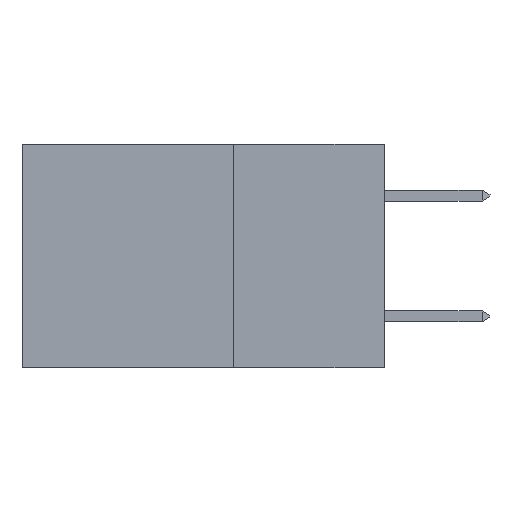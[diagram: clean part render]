
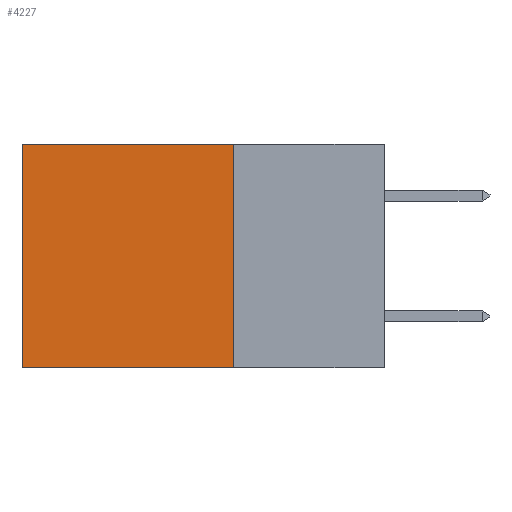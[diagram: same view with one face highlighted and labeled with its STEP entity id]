
A CAD part, left-side view. The second image highlights one B-rep face of the part: STEP entity #4227.
In plain terms, the highlighted planar face has unit normal (-1, 0, 0).
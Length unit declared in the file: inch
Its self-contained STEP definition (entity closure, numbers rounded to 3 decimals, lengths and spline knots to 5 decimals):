
#664 = LINE ( 'NONE', #10411, #8537 ) ;
#1403 = VERTEX_POINT ( 'NONE', #13510 ) ;
#2851 = DIRECTION ( 'NONE',  ( 0., 1., 0. ) ) ;
#2988 = VECTOR ( 'NONE', #2851, 39.37008 ) ;
#3219 = CARTESIAN_POINT ( 'NONE',  ( 0.2875, 0.25, -0.37 ) ) ;
#3693 = CARTESIAN_POINT ( 'NONE',  ( 0.2875, 0.6, -0.37 ) ) ;
#3797 = DIRECTION ( 'NONE',  ( 0., 0., -1. ) ) ;
#3848 = DIRECTION ( 'NONE',  ( 1., 0., 0. ) ) ;
#3862 = PLANE ( 'NONE',  #3937 ) ;
#3937 = AXIS2_PLACEMENT_3D ( 'NONE', #3963, #3848, #3797 ) ;
#3963 = CARTESIAN_POINT ( 'NONE',  ( 0.2875, 0.25, 0. ) ) ;
#3998 = EDGE_CURVE ( 'NONE', #10174, #11078, #10916, .T. ) ;
#4227 = ADVANCED_FACE ( 'NONE', ( #15307 ), #3862, .F. ) ;
#4277 = EDGE_CURVE ( 'NONE', #1403, #11078, #7198, .T. ) ;
#6881 = ORIENTED_EDGE ( 'NONE', *, *, #18691, .T. ) ;
#6943 = ORIENTED_EDGE ( 'NONE', *, *, #10071, .F. ) ;
#7198 = LINE ( 'NONE', #3219, #2988 ) ;
#7829 = DIRECTION ( 'NONE',  ( 0., 0., -1. ) ) ;
#7894 = CARTESIAN_POINT ( 'NONE',  ( 0.2875, 0.6, 0. ) ) ;
#8327 = VECTOR ( 'NONE', #18289, 39.37008 ) ;
#8537 = VECTOR ( 'NONE', #8934, 39.37008 ) ;
#8934 = DIRECTION ( 'NONE',  ( 0., 0., -1. ) ) ;
#9184 = CARTESIAN_POINT ( 'NONE',  ( 0.2875, 0.6, 0. ) ) ;
#10071 = EDGE_CURVE ( 'NONE', #13486, #1403, #664, .T. ) ;
#10174 = VERTEX_POINT ( 'NONE', #9184 ) ;
#10411 = CARTESIAN_POINT ( 'NONE',  ( 0.2875, 0.25, 0. ) ) ;
#10876 = ORIENTED_EDGE ( 'NONE', *, *, #4277, .F. ) ;
#10916 = LINE ( 'NONE', #7894, #17697 ) ;
#11078 = VERTEX_POINT ( 'NONE', #3693 ) ;
#13140 = CARTESIAN_POINT ( 'NONE',  ( 0.2875, 0.25, 0. ) ) ;
#13486 = VERTEX_POINT ( 'NONE', #17184 ) ;
#13510 = CARTESIAN_POINT ( 'NONE',  ( 0.2875, 0.25, -0.37 ) ) ;
#13814 = ORIENTED_EDGE ( 'NONE', *, *, #3998, .T. ) ;
#13905 = EDGE_LOOP ( 'NONE', ( #13814, #10876, #6943, #6881 ) ) ;
#15307 = FACE_OUTER_BOUND ( 'NONE', #13905, .T. ) ;
#15890 = LINE ( 'NONE', #13140, #8327 ) ;
#17184 = CARTESIAN_POINT ( 'NONE',  ( 0.2875, 0.25, 0. ) ) ;
#17697 = VECTOR ( 'NONE', #7829, 39.37008 ) ;
#18289 = DIRECTION ( 'NONE',  ( 0., 1., 0. ) ) ;
#18691 = EDGE_CURVE ( 'NONE', #13486, #10174, #15890, .T. ) ;
